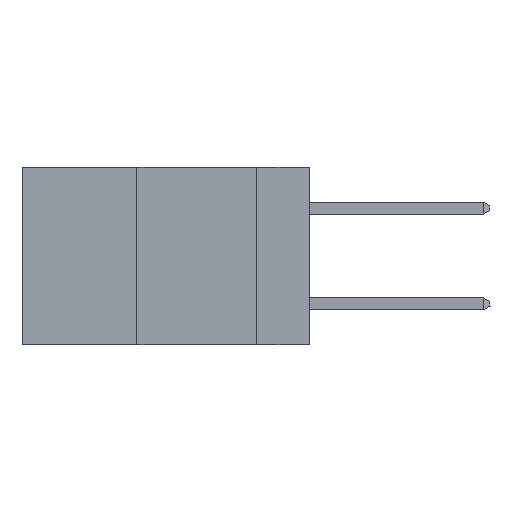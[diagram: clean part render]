
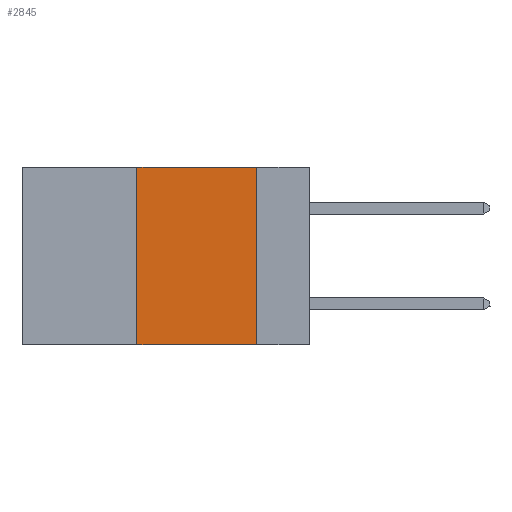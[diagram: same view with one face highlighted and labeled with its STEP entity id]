
A CAD part, left-side view. The second image highlights one B-rep face of the part: STEP entity #2845.
In plain terms, the highlighted planar face has unit normal (-1, 0, 0).
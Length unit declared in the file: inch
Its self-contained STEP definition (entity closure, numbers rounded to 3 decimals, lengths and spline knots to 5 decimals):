
#1697 = EDGE_CURVE ( 'NONE', #27712, #18020, #4178, .T. ) ;
#2845 = ADVANCED_FACE ( 'NONE', ( #27390 ), #8833, .F. ) ;
#3188 = DIRECTION ( 'NONE',  ( 0., 0., -1. ) ) ;
#3197 = EDGE_CURVE ( 'NONE', #18020, #20538, #30390, .T. ) ;
#4178 = LINE ( 'NONE', #14130, #29772 ) ;
#6165 = CARTESIAN_POINT ( 'NONE',  ( 0., 0.6, 0. ) ) ;
#6734 = ORIENTED_EDGE ( 'NONE', *, *, #3197, .F. ) ;
#6796 = DIRECTION ( 'NONE',  ( 0., -1., 0. ) ) ;
#8833 = PLANE ( 'NONE',  #10610 ) ;
#9674 = LINE ( 'NONE', #16782, #22790 ) ;
#10610 = AXIS2_PLACEMENT_3D ( 'NONE', #6165, #18242, #27882 ) ;
#11527 = CARTESIAN_POINT ( 'NONE',  ( 0., 0.11, -0.37 ) ) ;
#13025 = VECTOR ( 'NONE', #3188, 39.37008 ) ;
#13801 = ORIENTED_EDGE ( 'NONE', *, *, #1697, .F. ) ;
#14130 = CARTESIAN_POINT ( 'NONE',  ( 0., 0.6, 0. ) ) ;
#15060 = VECTOR ( 'NONE', #6796, 39.37008 ) ;
#16160 = CARTESIAN_POINT ( 'NONE',  ( 0., 0.11, 0. ) ) ;
#16782 = CARTESIAN_POINT ( 'NONE',  ( 0., 0.36, 0. ) ) ;
#17373 = ORIENTED_EDGE ( 'NONE', *, *, #27507, .F. ) ;
#17712 = EDGE_LOOP ( 'NONE', ( #6734, #13801, #17373, #18277 ) ) ;
#18020 = VERTEX_POINT ( 'NONE', #16160 ) ;
#18242 = DIRECTION ( 'NONE',  ( 1., 0., 0. ) ) ;
#18277 = ORIENTED_EDGE ( 'NONE', *, *, #28196, .T. ) ;
#19994 = CARTESIAN_POINT ( 'NONE',  ( 0., 0.11, 0. ) ) ;
#20538 = VERTEX_POINT ( 'NONE', #11527 ) ;
#22790 = VECTOR ( 'NONE', #28576, 39.37008 ) ;
#23760 = CARTESIAN_POINT ( 'NONE',  ( 0., 0.6, -0.37 ) ) ;
#24366 = CARTESIAN_POINT ( 'NONE',  ( 0., 0.36, 0. ) ) ;
#26447 = DIRECTION ( 'NONE',  ( 0., -1., 0. ) ) ;
#27277 = CARTESIAN_POINT ( 'NONE',  ( 0., 0.36, -0.37 ) ) ;
#27390 = FACE_OUTER_BOUND ( 'NONE', #17712, .T. ) ;
#27507 = EDGE_CURVE ( 'NONE', #31075, #27712, #9674, .T. ) ;
#27712 = VERTEX_POINT ( 'NONE', #24366 ) ;
#27882 = DIRECTION ( 'NONE',  ( 0., 0., -1. ) ) ;
#27939 = LINE ( 'NONE', #23760, #15060 ) ;
#28196 = EDGE_CURVE ( 'NONE', #31075, #20538, #27939, .T. ) ;
#28576 = DIRECTION ( 'NONE',  ( 0., 0., 1. ) ) ;
#29772 = VECTOR ( 'NONE', #26447, 39.37008 ) ;
#30390 = LINE ( 'NONE', #19994, #13025 ) ;
#31075 = VERTEX_POINT ( 'NONE', #27277 ) ;
